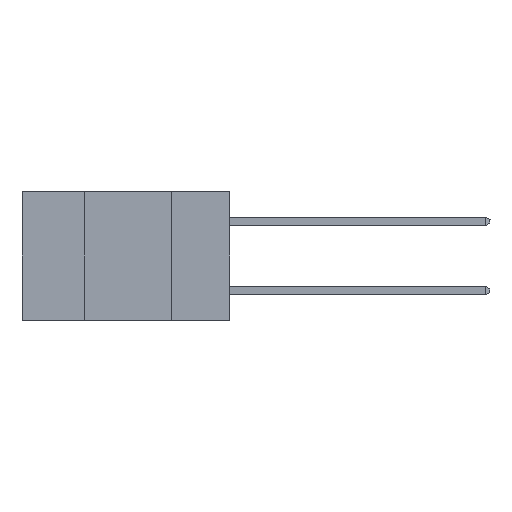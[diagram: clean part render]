
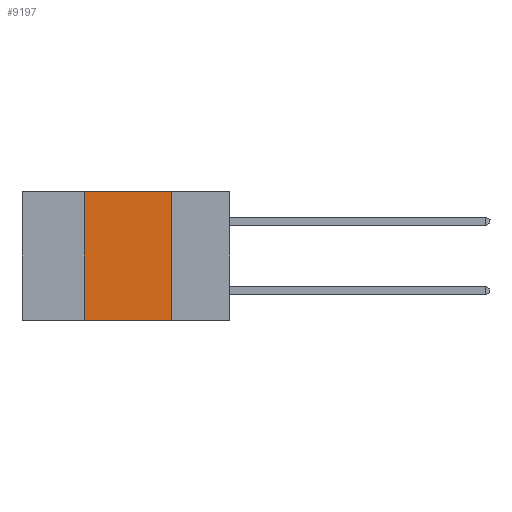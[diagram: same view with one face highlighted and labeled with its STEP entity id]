
A CAD part, left-side view. The second image highlights one B-rep face of the part: STEP entity #9197.
In plain terms, the highlighted planar face has unit normal (-1, 0, 0).
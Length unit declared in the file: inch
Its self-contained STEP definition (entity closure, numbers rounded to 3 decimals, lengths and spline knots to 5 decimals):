
#195 = LINE ( 'NONE', #1777, #17216 ) ;
#541 = VERTEX_POINT ( 'NONE', #15478 ) ;
#1475 = CARTESIAN_POINT ( 'NONE',  ( 0., 0.17, -0.37 ) ) ;
#1777 = CARTESIAN_POINT ( 'NONE',  ( 0., 0.6, -0.37 ) ) ;
#2157 = DIRECTION ( 'NONE',  ( 0., 0., -1. ) ) ;
#2725 = DIRECTION ( 'NONE',  ( 1., 0., 0. ) ) ;
#3091 = LINE ( 'NONE', #4396, #13809 ) ;
#4218 = DIRECTION ( 'NONE',  ( 0., 0., -1. ) ) ;
#4396 = CARTESIAN_POINT ( 'NONE',  ( 0., 0.6, 0. ) ) ;
#5129 = EDGE_CURVE ( 'NONE', #6782, #541, #3091, .T. ) ;
#5236 = VECTOR ( 'NONE', #17262, 39.37008 ) ;
#5541 = PLANE ( 'NONE',  #12136 ) ;
#6681 = ORIENTED_EDGE ( 'NONE', *, *, #12037, .F. ) ;
#6782 = VERTEX_POINT ( 'NONE', #13299 ) ;
#7022 = CARTESIAN_POINT ( 'NONE',  ( 0., 0.6, 0. ) ) ;
#8756 = CARTESIAN_POINT ( 'NONE',  ( 0., 0.42, -0.37 ) ) ;
#8965 = VERTEX_POINT ( 'NONE', #10601 ) ;
#9197 = ADVANCED_FACE ( 'NONE', ( #16671 ), #5541, .F. ) ;
#9298 = EDGE_CURVE ( 'NONE', #8965, #15018, #195, .T. ) ;
#10194 = DIRECTION ( 'NONE',  ( 0., -1., 0. ) ) ;
#10601 = CARTESIAN_POINT ( 'NONE',  ( 0., 0.42, -0.37 ) ) ;
#11044 = ORIENTED_EDGE ( 'NONE', *, *, #17239, .F. ) ;
#12037 = EDGE_CURVE ( 'NONE', #541, #15018, #16378, .T. ) ;
#12136 = AXIS2_PLACEMENT_3D ( 'NONE', #7022, #2725, #4218 ) ;
#12852 = VECTOR ( 'NONE', #2157, 39.37008 ) ;
#13299 = CARTESIAN_POINT ( 'NONE',  ( 0., 0.42, 0. ) ) ;
#13809 = VECTOR ( 'NONE', #14398, 39.37008 ) ;
#14344 = EDGE_LOOP ( 'NONE', ( #6681, #17822, #11044, #14555 ) ) ;
#14398 = DIRECTION ( 'NONE',  ( 0., -1., 0. ) ) ;
#14555 = ORIENTED_EDGE ( 'NONE', *, *, #9298, .T. ) ;
#14689 = CARTESIAN_POINT ( 'NONE',  ( 0., 0.17, -0.37 ) ) ;
#15018 = VERTEX_POINT ( 'NONE', #1475 ) ;
#15478 = CARTESIAN_POINT ( 'NONE',  ( 0., 0.17, 0. ) ) ;
#16378 = LINE ( 'NONE', #14689, #12852 ) ;
#16671 = FACE_OUTER_BOUND ( 'NONE', #14344, .T. ) ;
#17216 = VECTOR ( 'NONE', #10194, 39.37008 ) ;
#17239 = EDGE_CURVE ( 'NONE', #8965, #6782, #17705, .T. ) ;
#17262 = DIRECTION ( 'NONE',  ( 0., 0., 1. ) ) ;
#17705 = LINE ( 'NONE', #8756, #5236 ) ;
#17822 = ORIENTED_EDGE ( 'NONE', *, *, #5129, .F. ) ;
